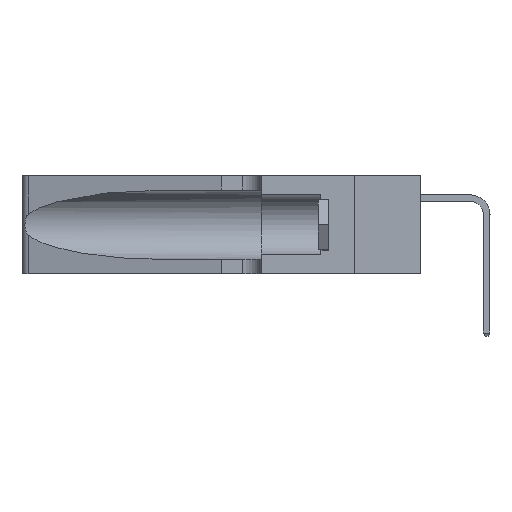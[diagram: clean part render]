
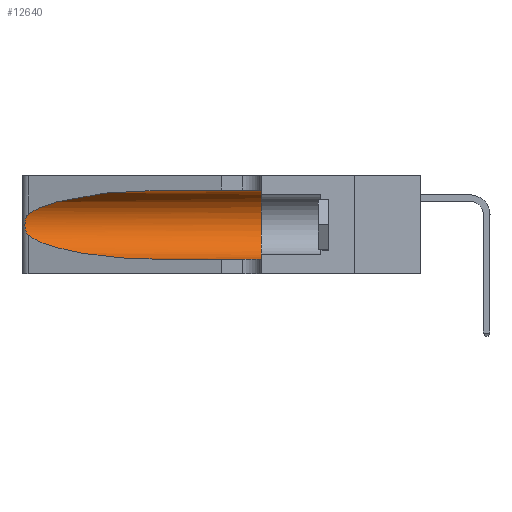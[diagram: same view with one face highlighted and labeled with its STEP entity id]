
A CAD part, left-side view. The second image highlights one B-rep face of the part: STEP entity #12640.
In plain terms, the highlighted cylindrical face has radius 3.308 mm (diameter 6.617 mm), a partial arc.
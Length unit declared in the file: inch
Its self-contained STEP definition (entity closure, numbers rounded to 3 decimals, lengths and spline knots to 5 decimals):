
#427 = VERTEX_POINT ( 'NONE', #2743 ) ;
#546 = ORIENTED_EDGE ( 'NONE', *, *, #18796, .F. ) ;
#597 = DIRECTION ( 'NONE',  ( 0., 0., 1. ) ) ;
#840 = CARTESIAN_POINT ( 'NONE',  ( 0.25789, 1.23486, 0.15765 ) ) ;
#1392 = CARTESIAN_POINT ( 'NONE',  ( 0.2373, 1.15595, 0.08982 ) ) ;
#1459 = ORIENTED_EDGE ( 'NONE', *, *, #17842, .T. ) ;
#1507 = EDGE_CURVE ( 'NONE', #17777, #427, #18391, .T. ) ;
#1526 = CARTESIAN_POINT ( 'NONE',  ( 0.1305, 0.72297, 0.31525 ) ) ;
#2317 = CARTESIAN_POINT ( 'NONE',  ( 0.1305, 1.61858, 0.31525 ) ) ;
#2407 = EDGE_CURVE ( 'NONE', #4416, #427, #18348, .T. ) ;
#2451 = CARTESIAN_POINT ( 'NONE',  ( 0.25555, 1.22993, 0.14849 ) ) ;
#2743 = CARTESIAN_POINT ( 'NONE',  ( 0.1305, 0.35, 0.05475 ) ) ;
#2802 = CARTESIAN_POINT ( 'NONE',  ( 0.1305, 1.61858, 0.185 ) ) ;
#2977 = CARTESIAN_POINT ( 'NONE',  ( 0.1305, 0.72297, 0.05475 ) ) ;
#2998 = CARTESIAN_POINT ( 'NONE',  ( 0.1305, 0.72297, 0.05475 ) ) ;
#3312 = B_SPLINE_CURVE_WITH_KNOTS ( 'NONE', 3,
 ( #17952, #19506, #14880, #5571, #16440, #7199, #18014, #8796, #19579, #10391, #840, #11911, #2451, #13429 ),
 .UNSPECIFIED., .F., .F.,
 ( 4, 2, 2, 2, 2, 2, 4 ),
 ( 0., 0.00027, 0.00053, 0.00107, 0.0016, 0.00187, 0.00214 ),
 .UNSPECIFIED. ) ;
#3364 = VERTEX_POINT ( 'NONE', #4505 ) ;
#4017 = AXIS2_PLACEMENT_3D ( 'NONE', #2802, #9148, #13782 ) ;
#4416 = VERTEX_POINT ( 'NONE', #11886 ) ;
#4505 = CARTESIAN_POINT ( 'NONE',  ( 0.1305, 0.72297, 0.31525 ) ) ;
#4641 = CARTESIAN_POINT ( 'NONE',  ( 0.1305, 1.61858, 0.05475 ) ) ;
#4648 = VERTEX_POINT ( 'NONE', #15510 ) ;
#5129 = ORIENTED_EDGE ( 'NONE', *, *, #2407, .F. ) ;
#5571 = CARTESIAN_POINT ( 'NONE',  ( 0.25787, 1.23484, 0.2124 ) ) ;
#5606 = EDGE_CURVE ( 'NONE', #11073, #4648, #3312, .T. ) ;
#6331 = CARTESIAN_POINT ( 'NONE',  ( 0.2373, 1.15595, 0.28018 ) ) ;
#6847 = CARTESIAN_POINT ( 'NONE',  ( 0.25487, 1.22718, 0.22369 ) ) ;
#6935 = VECTOR ( 'NONE', #14817, 39.37008 ) ;
#7199 = CARTESIAN_POINT ( 'NONE',  ( 0.26018, 1.23835, 0.19895 ) ) ;
#7564 = CYLINDRICAL_SURFACE ( 'NONE', #4017, 0.13025 ) ;
#8796 = CARTESIAN_POINT ( 'NONE',  ( 0.26075, 1.23896, 0.178 ) ) ;
#8801 = ORIENTED_EDGE ( 'NONE', *, *, #5606, .T. ) ;
#9148 = DIRECTION ( 'NONE',  ( 0., -1., 0. ) ) ;
#9693 = AXIS2_PLACEMENT_3D ( 'NONE', #19333, #10146, #597 ) ;
#9788 = ORIENTED_EDGE ( 'NONE', *, *, #1507, .T. ) ;
#10146 = DIRECTION ( 'NONE',  ( 0., 1., 0. ) ) ;
#10391 = CARTESIAN_POINT ( 'NONE',  ( 0.25856, 1.23593, 0.16098 ) ) ;
#10921 = CARTESIAN_POINT ( 'NONE',  ( 0.25487, 1.22718, 0.14631 ) ) ;
#11029 = CARTESIAN_POINT ( 'NONE',  ( 0.18966, 0.96281, 0.31525 ) ) ;
#11073 = VERTEX_POINT ( 'NONE', #6847 ) ;
#11886 = CARTESIAN_POINT ( 'NONE',  ( 0.1305, 0.35, 0.31525 ) ) ;
#11911 = CARTESIAN_POINT ( 'NONE',  ( 0.25639, 1.23186, 0.15144 ) ) ;
#12444 = CARTESIAN_POINT ( 'NONE',  ( 0.18966, 0.96281, 0.05475 ) ) ;
#12640 = ADVANCED_FACE ( 'NONE', ( #15751 ), #7564, .F. ) ;
#13429 = CARTESIAN_POINT ( 'NONE',  ( 0.25487, 1.22718, 0.14631 ) ) ;
#13782 = DIRECTION ( 'NONE',  ( 0., 0., -1. ) ) ;
#14080 =( BOUNDED_CURVE ( )  B_SPLINE_CURVE ( 3, ( #10921, #1392, #12444, #2998 ),
 .UNSPECIFIED., .F., .F. ) 
 B_SPLINE_CURVE_WITH_KNOTS ( ( 4, 4 ),
 ( 3.44316, 4.71239 ),
 .UNSPECIFIED. ) 
 CURVE ( )  GEOMETRIC_REPRESENTATION_ITEM ( )  RATIONAL_B_SPLINE_CURVE ( ( 1., 0.87, 0.87, 1. ) ) 
 REPRESENTATION_ITEM ( '' )  );
#14467 = EDGE_LOOP ( 'NONE', ( #1459, #8801, #14671, #9788, #5129, #546 ) ) ;
#14671 = ORIENTED_EDGE ( 'NONE', *, *, #17142, .T. ) ;
#14817 = DIRECTION ( 'NONE',  ( 0., -1., 0. ) ) ;
#14880 = CARTESIAN_POINT ( 'NONE',  ( 0.25639, 1.23184, 0.21858 ) ) ;
#15510 = CARTESIAN_POINT ( 'NONE',  ( 0.25487, 1.22718, 0.14631 ) ) ;
#15751 = FACE_OUTER_BOUND ( 'NONE', #14467, .T. ) ;
#16440 = CARTESIAN_POINT ( 'NONE',  ( 0.25854, 1.2359, 0.20912 ) ) ;
#17101 = DIRECTION ( 'NONE',  ( 0., -1., 0. ) ) ;
#17142 = EDGE_CURVE ( 'NONE', #4648, #17777, #14080, .T. ) ;
#17164 = CARTESIAN_POINT ( 'NONE',  ( 0.25487, 1.22718, 0.22369 ) ) ;
#17777 = VERTEX_POINT ( 'NONE', #2977 ) ;
#17842 = EDGE_CURVE ( 'NONE', #3364, #11073, #19779, .T. ) ;
#17902 = VECTOR ( 'NONE', #17101, 39.37008 ) ;
#17952 = CARTESIAN_POINT ( 'NONE',  ( 0.25487, 1.22718, 0.22369 ) ) ;
#18014 = CARTESIAN_POINT ( 'NONE',  ( 0.26075, 1.23896, 0.19203 ) ) ;
#18348 = CIRCLE ( 'NONE', #9693, 0.13025 ) ;
#18391 = LINE ( 'NONE', #4641, #17902 ) ;
#18796 = EDGE_CURVE ( 'NONE', #3364, #4416, #19289, .T. ) ;
#19289 = LINE ( 'NONE', #2317, #6935 ) ;
#19333 = CARTESIAN_POINT ( 'NONE',  ( 0.1305, 0.35, 0.185 ) ) ;
#19506 = CARTESIAN_POINT ( 'NONE',  ( 0.25555, 1.22994, 0.2215 ) ) ;
#19579 = CARTESIAN_POINT ( 'NONE',  ( 0.26017, 1.23833, 0.17102 ) ) ;
#19779 =( BOUNDED_CURVE ( )  B_SPLINE_CURVE ( 3, ( #1526, #11029, #6331, #17164 ),
 .UNSPECIFIED., .F., .F. ) 
 B_SPLINE_CURVE_WITH_KNOTS ( ( 4, 4 ),
 ( 1.5708, 2.84003 ),
 .UNSPECIFIED. ) 
 CURVE ( )  GEOMETRIC_REPRESENTATION_ITEM ( )  RATIONAL_B_SPLINE_CURVE ( ( 1., 0.87, 0.87, 1. ) ) 
 REPRESENTATION_ITEM ( '' )  );
